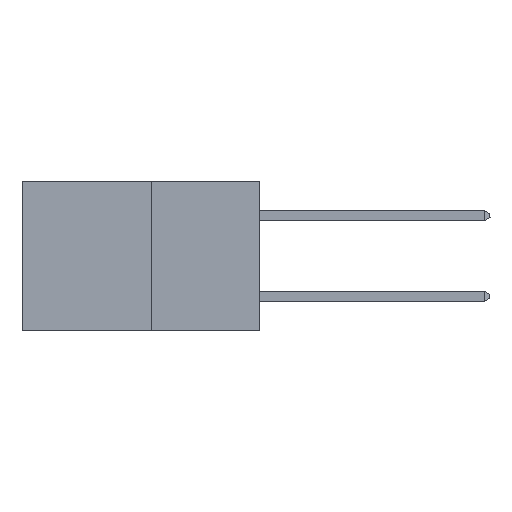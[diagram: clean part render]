
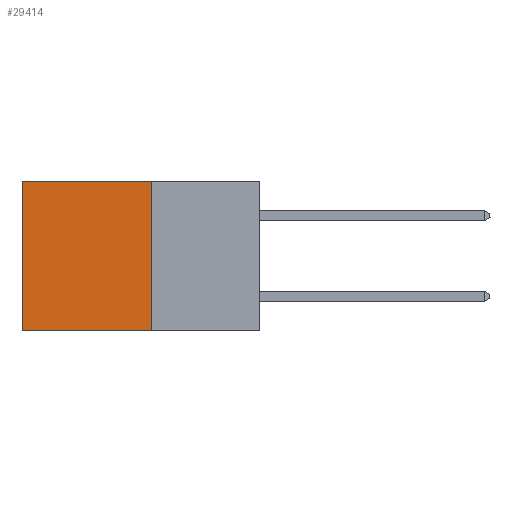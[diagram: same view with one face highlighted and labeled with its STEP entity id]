
A CAD part, left-side view. The second image highlights one B-rep face of the part: STEP entity #29414.
In plain terms, the highlighted planar face has unit normal (-1, 0, 0).
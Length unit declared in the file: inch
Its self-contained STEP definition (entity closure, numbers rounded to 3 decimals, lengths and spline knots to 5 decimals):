
#2513 = LINE ( 'NONE', #21464, #29729 ) ;
#3253 = EDGE_CURVE ( 'NONE', #9848, #30698, #21101, .T. ) ;
#3297 = DIRECTION ( 'NONE',  ( 0., 1., 0. ) ) ;
#5108 = LINE ( 'NONE', #27682, #33089 ) ;
#5783 = VECTOR ( 'NONE', #7526, 39.37008 ) ;
#5933 = EDGE_CURVE ( 'NONE', #30698, #6961, #2513, .T. ) ;
#6961 = VERTEX_POINT ( 'NONE', #9299 ) ;
#7526 = DIRECTION ( 'NONE',  ( 0., 1., 0. ) ) ;
#7903 = DIRECTION ( 'NONE',  ( 0., 0., -1. ) ) ;
#8429 = ORIENTED_EDGE ( 'NONE', *, *, #3253, .T. ) ;
#9299 = CARTESIAN_POINT ( 'NONE',  ( 0.277, 0.59, -0.37 ) ) ;
#9848 = VERTEX_POINT ( 'NONE', #21236 ) ;
#10122 = FACE_OUTER_BOUND ( 'NONE', #16314, .T. ) ;
#10457 = LINE ( 'NONE', #29569, #16857 ) ;
#12510 = CARTESIAN_POINT ( 'NONE',  ( 0.277, 0.27, -0.37 ) ) ;
#13142 = EDGE_CURVE ( 'NONE', #9848, #30513, #10457, .T. ) ;
#16277 = CARTESIAN_POINT ( 'NONE',  ( 0.277, 0.27, -0.37 ) ) ;
#16314 = EDGE_LOOP ( 'NONE', ( #29688, #19418, #20617, #8429 ) ) ;
#16857 = VECTOR ( 'NONE', #7903, 39.37008 ) ;
#19006 = DIRECTION ( 'NONE',  ( 0., 0., -1. ) ) ;
#19418 = ORIENTED_EDGE ( 'NONE', *, *, #28276, .F. ) ;
#20617 = ORIENTED_EDGE ( 'NONE', *, *, #13142, .F. ) ;
#21101 = LINE ( 'NONE', #26087, #5783 ) ;
#21236 = CARTESIAN_POINT ( 'NONE',  ( 0.277, 0.27, 0. ) ) ;
#21464 = CARTESIAN_POINT ( 'NONE',  ( 0.277, 0.59, -0.37 ) ) ;
#26087 = CARTESIAN_POINT ( 'NONE',  ( 0.277, 0.27, 0. ) ) ;
#26874 = DIRECTION ( 'NONE',  ( 0., 0., -1. ) ) ;
#27682 = CARTESIAN_POINT ( 'NONE',  ( 0.277, 0.27, -0.37 ) ) ;
#28276 = EDGE_CURVE ( 'NONE', #30513, #6961, #5108, .T. ) ;
#29414 = ADVANCED_FACE ( 'NONE', ( #10122 ), #32462, .F. ) ;
#29419 = CARTESIAN_POINT ( 'NONE',  ( 0.277, 0.59, 0. ) ) ;
#29569 = CARTESIAN_POINT ( 'NONE',  ( 0.277, 0.27, -0.37 ) ) ;
#29688 = ORIENTED_EDGE ( 'NONE', *, *, #5933, .T. ) ;
#29729 = VECTOR ( 'NONE', #26874, 39.37008 ) ;
#29739 = AXIS2_PLACEMENT_3D ( 'NONE', #16277, #35206, #19006 ) ;
#30513 = VERTEX_POINT ( 'NONE', #12510 ) ;
#30698 = VERTEX_POINT ( 'NONE', #29419 ) ;
#32462 = PLANE ( 'NONE',  #29739 ) ;
#33089 = VECTOR ( 'NONE', #3297, 39.37008 ) ;
#35206 = DIRECTION ( 'NONE',  ( 1., 0., 0. ) ) ;
